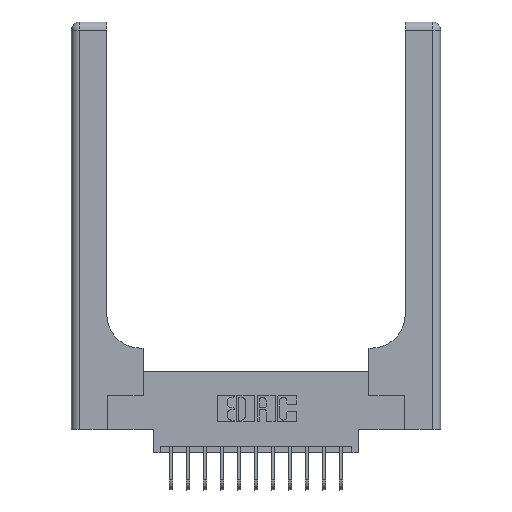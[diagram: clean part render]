
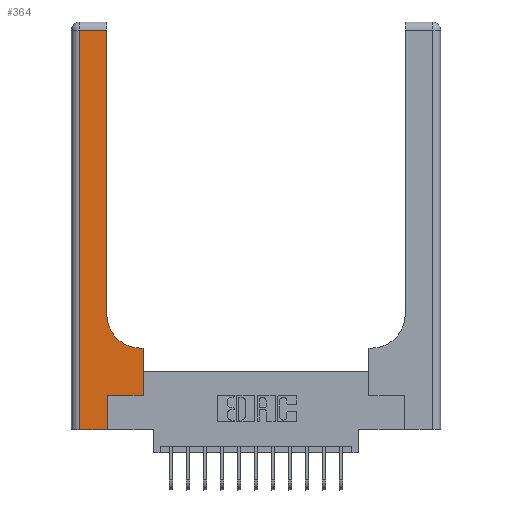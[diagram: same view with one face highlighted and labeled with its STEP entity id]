
A CAD part, top view. The second image highlights one B-rep face of the part: STEP entity #364.
In plain terms, the highlighted planar face has unit normal (0, 0, 1).
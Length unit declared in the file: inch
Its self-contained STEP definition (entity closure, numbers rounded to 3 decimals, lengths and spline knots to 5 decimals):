
#364 = ADVANCED_FACE ( 'NONE', ( #12472 ), #12582, .F. ) ;
#629 = VECTOR ( 'NONE', #11220, 39.37008 ) ;
#695 = ORIENTED_EDGE ( 'NONE', *, *, #15856, .T. ) ;
#885 = CARTESIAN_POINT ( 'NONE',  ( 0.06, 0., 0.37 ) ) ;
#1109 = VERTEX_POINT ( 'NONE', #4108 ) ;
#1110 = ORIENTED_EDGE ( 'NONE', *, *, #13082, .T. ) ;
#1184 = DIRECTION ( 'NONE',  ( 1., 0., 0. ) ) ;
#1185 = DIRECTION ( 'NONE',  ( -1., 0., 0. ) ) ;
#1680 = VECTOR ( 'NONE', #6498, 39.37008 ) ;
#2350 = ORIENTED_EDGE ( 'NONE', *, *, #10218, .T. ) ;
#2768 = VECTOR ( 'NONE', #7186, 39.37008 ) ;
#2942 = CARTESIAN_POINT ( 'NONE',  ( 0.06, 3., 0.37 ) ) ;
#3410 = CARTESIAN_POINT ( 'NONE',  ( 0.265, 0., 0.37 ) ) ;
#3474 = EDGE_CURVE ( 'NONE', #11176, #8003, #4077, .T. ) ;
#3621 = EDGE_CURVE ( 'NONE', #11381, #11176, #15487, .T. ) ;
#3654 = VERTEX_POINT ( 'NONE', #4540 ) ;
#3963 = CARTESIAN_POINT ( 'NONE',  ( 0.26, 3., 0.37 ) ) ;
#4077 = LINE ( 'NONE', #9301, #10404 ) ;
#4082 = EDGE_CURVE ( 'NONE', #11897, #8922, #9049, .T. ) ;
#4108 = CARTESIAN_POINT ( 'NONE',  ( 0.26, 0.85, 0.37 ) ) ;
#4540 = CARTESIAN_POINT ( 'NONE',  ( 0.265, 0., 0.37 ) ) ;
#4560 = ORIENTED_EDGE ( 'NONE', *, *, #10145, .T. ) ;
#4967 = ORIENTED_EDGE ( 'NONE', *, *, #3474, .T. ) ;
#5125 = LINE ( 'NONE', #3963, #1680 ) ;
#5769 = EDGE_CURVE ( 'NONE', #5782, #11897, #8409, .T. ) ;
#5782 = VERTEX_POINT ( 'NONE', #7511 ) ;
#6184 = LINE ( 'NONE', #3410, #2768 ) ;
#6233 = CARTESIAN_POINT ( 'NONE',  ( 0., 2.94, 0.37 ) ) ;
#6498 = DIRECTION ( 'NONE',  ( 0., 1., 0. ) ) ;
#6656 = CIRCLE ( 'NONE', #7416, 0.25 ) ;
#6716 = ORIENTED_EDGE ( 'NONE', *, *, #5769, .T. ) ;
#6748 = CARTESIAN_POINT ( 'NONE',  ( 0.528, 0.6, 0.37 ) ) ;
#7114 = ORIENTED_EDGE ( 'NONE', *, *, #4082, .T. ) ;
#7186 = DIRECTION ( 'NONE',  ( 0., 1., 0. ) ) ;
#7416 = AXIS2_PLACEMENT_3D ( 'NONE', #16334, #8864, #1184 ) ;
#7511 = CARTESIAN_POINT ( 'NONE',  ( 0.26, 2.94, 0.37 ) ) ;
#7935 = ORIENTED_EDGE ( 'NONE', *, *, #3621, .T. ) ;
#7941 = CARTESIAN_POINT ( 'NONE',  ( 0., 0., 0.37 ) ) ;
#8003 = VERTEX_POINT ( 'NONE', #13335 ) ;
#8409 = LINE ( 'NONE', #6233, #11722 ) ;
#8534 = ORIENTED_EDGE ( 'NONE', *, *, #15158, .T. ) ;
#8853 = VECTOR ( 'NONE', #12027, 39.37008 ) ;
#8864 = DIRECTION ( 'NONE',  ( 0., 0., -1. ) ) ;
#8865 = DIRECTION ( 'NONE',  ( 0., 0., -1. ) ) ;
#8922 = VERTEX_POINT ( 'NONE', #885 ) ;
#8965 = CARTESIAN_POINT ( 'NONE',  ( 0.265, 0.25, 0.37 ) ) ;
#9049 = LINE ( 'NONE', #2942, #15312 ) ;
#9301 = CARTESIAN_POINT ( 'NONE',  ( 0.26, 0.6, 0.37 ) ) ;
#9862 = EDGE_LOOP ( 'NONE', ( #8534, #6716, #7114, #695, #1110, #4560, #7935, #4967, #2350 ) ) ;
#9956 = CARTESIAN_POINT ( 'NONE',  ( 0.265, 0.25, 0.37 ) ) ;
#10145 = EDGE_CURVE ( 'NONE', #15108, #11381, #14150, .T. ) ;
#10218 = EDGE_CURVE ( 'NONE', #8003, #1109, #6656, .T. ) ;
#10404 = VECTOR ( 'NONE', #15532, 39.37008 ) ;
#11176 = VERTEX_POINT ( 'NONE', #6748 ) ;
#11220 = DIRECTION ( 'NONE',  ( 1., 0., 0. ) ) ;
#11381 = VERTEX_POINT ( 'NONE', #15854 ) ;
#11603 = VECTOR ( 'NONE', #12908, 39.37008 ) ;
#11722 = VECTOR ( 'NONE', #15040, 39.37008 ) ;
#11897 = VERTEX_POINT ( 'NONE', #13260 ) ;
#12027 = DIRECTION ( 'NONE',  ( 0., 1., 0. ) ) ;
#12472 = FACE_OUTER_BOUND ( 'NONE', #9862, .T. ) ;
#12582 = PLANE ( 'NONE',  #14045 ) ;
#12908 = DIRECTION ( 'NONE',  ( 1., 0., 0. ) ) ;
#13049 = DIRECTION ( 'NONE',  ( 0., -1., 0. ) ) ;
#13082 = EDGE_CURVE ( 'NONE', #3654, #15108, #6184, .T. ) ;
#13260 = CARTESIAN_POINT ( 'NONE',  ( 0.06, 2.94, 0.37 ) ) ;
#13335 = CARTESIAN_POINT ( 'NONE',  ( 0.51, 0.6, 0.37 ) ) ;
#14045 = AXIS2_PLACEMENT_3D ( 'NONE', #15102, #8865, #1185 ) ;
#14150 = LINE ( 'NONE', #9956, #629 ) ;
#14557 = CARTESIAN_POINT ( 'NONE',  ( 0.528, 0.25, 0.37 ) ) ;
#15040 = DIRECTION ( 'NONE',  ( -1., 0., 0. ) ) ;
#15102 = CARTESIAN_POINT ( 'NONE',  ( 0., 3., 0.37 ) ) ;
#15108 = VERTEX_POINT ( 'NONE', #8965 ) ;
#15158 = EDGE_CURVE ( 'NONE', #1109, #5782, #5125, .T. ) ;
#15312 = VECTOR ( 'NONE', #13049, 39.37008 ) ;
#15326 = LINE ( 'NONE', #7941, #11603 ) ;
#15487 = LINE ( 'NONE', #14557, #8853 ) ;
#15532 = DIRECTION ( 'NONE',  ( -1., 0., 0. ) ) ;
#15854 = CARTESIAN_POINT ( 'NONE',  ( 0.528, 0.25, 0.37 ) ) ;
#15856 = EDGE_CURVE ( 'NONE', #8922, #3654, #15326, .T. ) ;
#16334 = CARTESIAN_POINT ( 'NONE',  ( 0.51, 0.85, 0.37 ) ) ;
